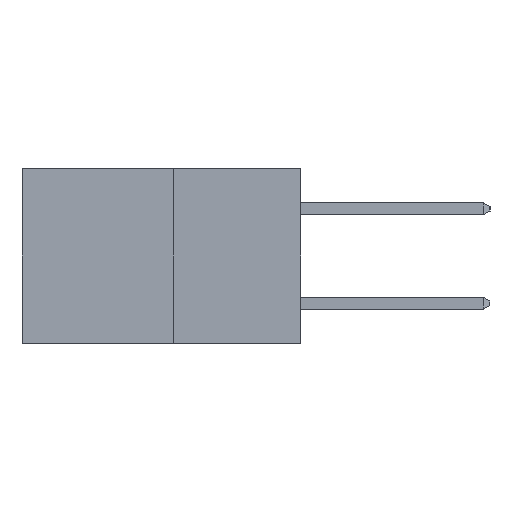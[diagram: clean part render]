
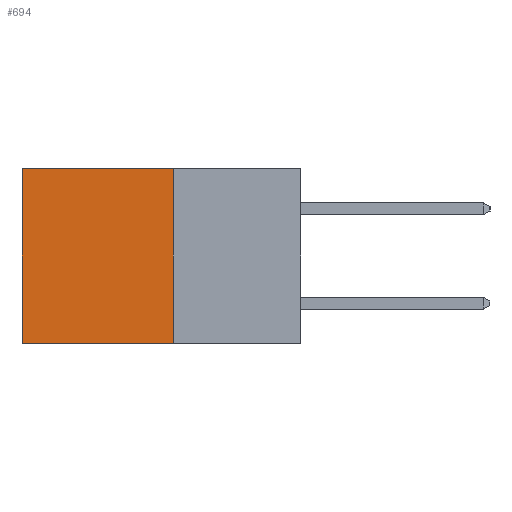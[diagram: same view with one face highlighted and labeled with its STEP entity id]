
A CAD part, left-side view. The second image highlights one B-rep face of the part: STEP entity #694.
In plain terms, the highlighted planar face has unit normal (-1, 0, 0).
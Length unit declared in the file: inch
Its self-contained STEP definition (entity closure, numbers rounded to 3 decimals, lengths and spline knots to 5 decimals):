
#168 = DIRECTION ( 'NONE',  ( 0., 0., -1. ) ) ;
#199 = EDGE_CURVE ( 'NONE', #8209, #4554, #8742, .T. ) ;
#694 = ADVANCED_FACE ( 'NONE', ( #6557 ), #9866, .F. ) ;
#1036 = ORIENTED_EDGE ( 'NONE', *, *, #1674, .F. ) ;
#1341 = DIRECTION ( 'NONE',  ( 0., 0., -1. ) ) ;
#1674 = EDGE_CURVE ( 'NONE', #4554, #11549, #8708, .T. ) ;
#2184 = CARTESIAN_POINT ( 'NONE',  ( 0.277, 0.27, 0. ) ) ;
#2330 = DIRECTION ( 'NONE',  ( 0., 1., 0. ) ) ;
#2562 = VECTOR ( 'NONE', #168, 39.37008 ) ;
#3184 = ORIENTED_EDGE ( 'NONE', *, *, #5065, .T. ) ;
#3280 = DIRECTION ( 'NONE',  ( 1., 0., 0. ) ) ;
#3491 = CARTESIAN_POINT ( 'NONE',  ( 0.277, 0.27, -0.37 ) ) ;
#3597 = VECTOR ( 'NONE', #6838, 39.37008 ) ;
#4554 = VERTEX_POINT ( 'NONE', #3491 ) ;
#4934 = CARTESIAN_POINT ( 'NONE',  ( 0.277, 0.59, -0.37 ) ) ;
#4977 = CARTESIAN_POINT ( 'NONE',  ( 0.277, 0.59, 0. ) ) ;
#5031 = LINE ( 'NONE', #10459, #2562 ) ;
#5065 = EDGE_CURVE ( 'NONE', #8209, #6626, #8169, .T. ) ;
#5164 = CARTESIAN_POINT ( 'NONE',  ( 0.277, 0.27, -0.37 ) ) ;
#5711 = CARTESIAN_POINT ( 'NONE',  ( 0.277, 0.27, -0.37 ) ) ;
#5768 = CARTESIAN_POINT ( 'NONE',  ( 0.277, 0.27, -0.37 ) ) ;
#6253 = VECTOR ( 'NONE', #2330, 39.37008 ) ;
#6282 = VECTOR ( 'NONE', #10482, 39.37008 ) ;
#6557 = FACE_OUTER_BOUND ( 'NONE', #10920, .T. ) ;
#6626 = VERTEX_POINT ( 'NONE', #4977 ) ;
#6838 = DIRECTION ( 'NONE',  ( 0., 1., 0. ) ) ;
#7004 = CARTESIAN_POINT ( 'NONE',  ( 0.277, 0.27, 0. ) ) ;
#7760 = AXIS2_PLACEMENT_3D ( 'NONE', #5164, #3280, #1341 ) ;
#8169 = LINE ( 'NONE', #7004, #3597 ) ;
#8209 = VERTEX_POINT ( 'NONE', #2184 ) ;
#8708 = LINE ( 'NONE', #5711, #6253 ) ;
#8742 = LINE ( 'NONE', #5768, #6282 ) ;
#9345 = ORIENTED_EDGE ( 'NONE', *, *, #199, .F. ) ;
#9740 = EDGE_CURVE ( 'NONE', #6626, #11549, #5031, .T. ) ;
#9866 = PLANE ( 'NONE',  #7760 ) ;
#10342 = ORIENTED_EDGE ( 'NONE', *, *, #9740, .T. ) ;
#10459 = CARTESIAN_POINT ( 'NONE',  ( 0.277, 0.59, -0.37 ) ) ;
#10482 = DIRECTION ( 'NONE',  ( 0., 0., -1. ) ) ;
#10920 = EDGE_LOOP ( 'NONE', ( #10342, #1036, #9345, #3184 ) ) ;
#11549 = VERTEX_POINT ( 'NONE', #4934 ) ;
